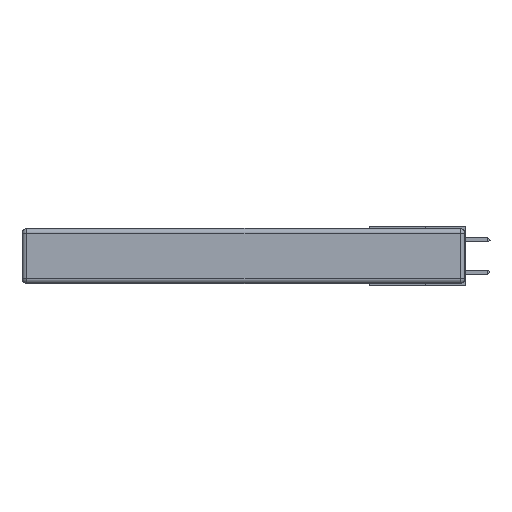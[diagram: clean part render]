
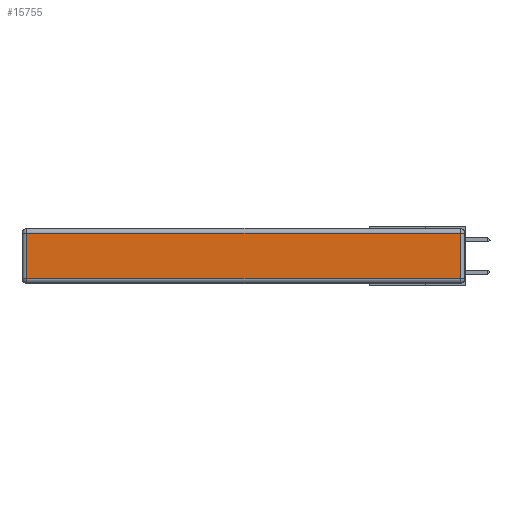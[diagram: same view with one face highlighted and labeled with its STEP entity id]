
A CAD part, left-side view. The second image highlights one B-rep face of the part: STEP entity #15755.
In plain terms, the highlighted planar face has unit normal (-1, 0, 0).
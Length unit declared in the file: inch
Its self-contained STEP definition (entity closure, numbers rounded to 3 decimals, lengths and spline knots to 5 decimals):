
#410 = VERTEX_POINT ( 'NONE', #18432 ) ;
#1071 = DIRECTION ( 'NONE',  ( 0., 0., -1. ) ) ;
#1557 = LINE ( 'NONE', #19380, #4091 ) ;
#2057 = PLANE ( 'NONE',  #3927 ) ;
#2361 = ORIENTED_EDGE ( 'NONE', *, *, #18653, .T. ) ;
#2920 = VERTEX_POINT ( 'NONE', #8636 ) ;
#2985 = DIRECTION ( 'NONE',  ( 0., 0., 1. ) ) ;
#3595 = CARTESIAN_POINT ( 'NONE',  ( 0., 2.75, -0.03 ) ) ;
#3927 = AXIS2_PLACEMENT_3D ( 'NONE', #20460, #13917, #22828 ) ;
#4091 = VECTOR ( 'NONE', #19780, 39.37008 ) ;
#4674 = LINE ( 'NONE', #14988, #5391 ) ;
#4769 = EDGE_CURVE ( 'NONE', #13777, #21186, #1557, .T. ) ;
#5391 = VECTOR ( 'NONE', #1071, 39.37008 ) ;
#5984 = VECTOR ( 'NONE', #10707, 39.37008 ) ;
#7749 = CARTESIAN_POINT ( 'NONE',  ( 0., 0.03, -0.343 ) ) ;
#7975 = FACE_OUTER_BOUND ( 'NONE', #29694, .T. ) ;
#8636 = CARTESIAN_POINT ( 'NONE',  ( 0., 2.72, -0.03 ) ) ;
#10707 = DIRECTION ( 'NONE',  ( 0., 1., 0. ) ) ;
#12144 = LINE ( 'NONE', #7749, #23108 ) ;
#13777 = VERTEX_POINT ( 'NONE', #28438 ) ;
#13917 = DIRECTION ( 'NONE',  ( -1., 0., 0. ) ) ;
#14988 = CARTESIAN_POINT ( 'NONE',  ( 0., 2.72, -0.343 ) ) ;
#15755 = ADVANCED_FACE ( 'NONE', ( #7975 ), #2057, .T. ) ;
#16757 = ORIENTED_EDGE ( 'NONE', *, *, #28415, .T. ) ;
#16842 = LINE ( 'NONE', #3595, #5984 ) ;
#18432 = CARTESIAN_POINT ( 'NONE',  ( 0., 0.03, -0.03 ) ) ;
#18653 = EDGE_CURVE ( 'NONE', #21186, #410, #12144, .T. ) ;
#18761 = ORIENTED_EDGE ( 'NONE', *, *, #4769, .T. ) ;
#19380 = CARTESIAN_POINT ( 'NONE',  ( 0., 0., -0.313 ) ) ;
#19780 = DIRECTION ( 'NONE',  ( 0., -1., 0. ) ) ;
#20460 = CARTESIAN_POINT ( 'NONE',  ( 0., 0., -0.343 ) ) ;
#21186 = VERTEX_POINT ( 'NONE', #22153 ) ;
#22153 = CARTESIAN_POINT ( 'NONE',  ( 0., 0.03, -0.313 ) ) ;
#22828 = DIRECTION ( 'NONE',  ( 0., 0., 1. ) ) ;
#23108 = VECTOR ( 'NONE', #2985, 39.37008 ) ;
#25634 = EDGE_CURVE ( 'NONE', #2920, #13777, #4674, .T. ) ;
#25838 = ORIENTED_EDGE ( 'NONE', *, *, #25634, .T. ) ;
#28415 = EDGE_CURVE ( 'NONE', #410, #2920, #16842, .T. ) ;
#28438 = CARTESIAN_POINT ( 'NONE',  ( 0., 2.72, -0.313 ) ) ;
#29694 = EDGE_LOOP ( 'NONE', ( #18761, #2361, #16757, #25838 ) ) ;
